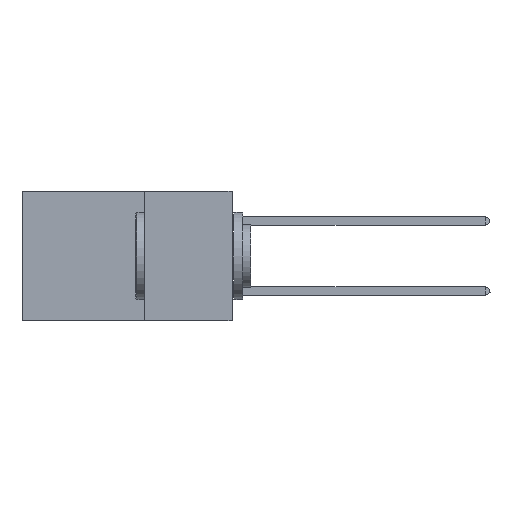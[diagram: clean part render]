
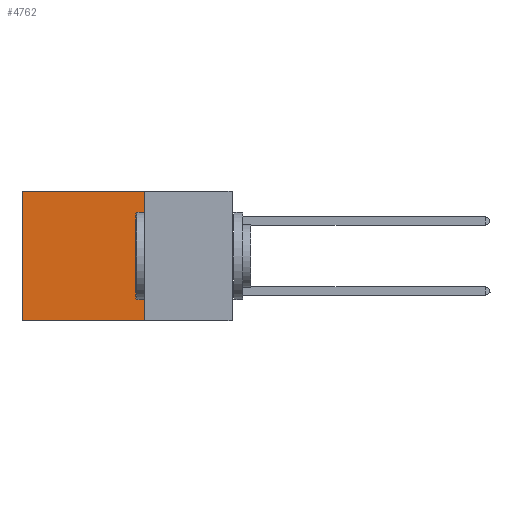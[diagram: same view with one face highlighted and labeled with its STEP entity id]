
A CAD part, left-side view. The second image highlights one B-rep face of the part: STEP entity #4762.
In plain terms, the highlighted planar face has unit normal (-1, 0, 0).
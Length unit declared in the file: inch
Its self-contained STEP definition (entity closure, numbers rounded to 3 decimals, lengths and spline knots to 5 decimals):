
#430 = VECTOR ( 'NONE', #8802, 39.37008 ) ;
#1242 = LINE ( 'NONE', #15329, #17716 ) ;
#1380 = DIRECTION ( 'NONE',  ( 0., 1., 0. ) ) ;
#1660 = DIRECTION ( 'NONE',  ( 0., 0., -1. ) ) ;
#2346 = CARTESIAN_POINT ( 'NONE',  ( 0.2875, 0.6, 0. ) ) ;
#2479 = ORIENTED_EDGE ( 'NONE', *, *, #14017, .T. ) ;
#4374 = CARTESIAN_POINT ( 'NONE',  ( 0.2875, 0.6, -0.37 ) ) ;
#4662 = AXIS2_PLACEMENT_3D ( 'NONE', #23682, #25618, #19471 ) ;
#4762 = ADVANCED_FACE ( 'NONE', ( #19505 ), #15583, .F. ) ;
#5738 = EDGE_CURVE ( 'NONE', #18091, #20064, #22649, .T. ) ;
#6403 = ORIENTED_EDGE ( 'NONE', *, *, #22559, .T. ) ;
#8564 = LINE ( 'NONE', #21800, #10503 ) ;
#8802 = DIRECTION ( 'NONE',  ( 0., 0., -1. ) ) ;
#10503 = VECTOR ( 'NONE', #1660, 39.37008 ) ;
#11326 = ORIENTED_EDGE ( 'NONE', *, *, #24099, .F. ) ;
#14017 = EDGE_CURVE ( 'NONE', #19456, #25180, #8564, .T. ) ;
#14336 = ORIENTED_EDGE ( 'NONE', *, *, #5738, .F. ) ;
#15314 = EDGE_LOOP ( 'NONE', ( #2479, #11326, #14336, #6403 ) ) ;
#15329 = CARTESIAN_POINT ( 'NONE',  ( 0.2875, 0.25, 0. ) ) ;
#15583 = PLANE ( 'NONE',  #4662 ) ;
#17716 = VECTOR ( 'NONE', #25544, 39.37008 ) ;
#18091 = VERTEX_POINT ( 'NONE', #20521 ) ;
#19456 = VERTEX_POINT ( 'NONE', #2346 ) ;
#19471 = DIRECTION ( 'NONE',  ( 0., 0., -1. ) ) ;
#19505 = FACE_OUTER_BOUND ( 'NONE', #15314, .T. ) ;
#20064 = VERTEX_POINT ( 'NONE', #23119 ) ;
#20521 = CARTESIAN_POINT ( 'NONE',  ( 0.2875, 0.25, 0. ) ) ;
#21800 = CARTESIAN_POINT ( 'NONE',  ( 0.2875, 0.6, 0. ) ) ;
#22106 = VECTOR ( 'NONE', #1380, 39.37008 ) ;
#22559 = EDGE_CURVE ( 'NONE', #18091, #19456, #1242, .T. ) ;
#22649 = LINE ( 'NONE', #23114, #430 ) ;
#23114 = CARTESIAN_POINT ( 'NONE',  ( 0.2875, 0.25, 0. ) ) ;
#23119 = CARTESIAN_POINT ( 'NONE',  ( 0.2875, 0.25, -0.37 ) ) ;
#23376 = CARTESIAN_POINT ( 'NONE',  ( 0.2875, 0.25, -0.37 ) ) ;
#23682 = CARTESIAN_POINT ( 'NONE',  ( 0.2875, 0.25, 0. ) ) ;
#24099 = EDGE_CURVE ( 'NONE', #20064, #25180, #24929, .T. ) ;
#24929 = LINE ( 'NONE', #23376, #22106 ) ;
#25180 = VERTEX_POINT ( 'NONE', #4374 ) ;
#25544 = DIRECTION ( 'NONE',  ( 0., 1., 0. ) ) ;
#25618 = DIRECTION ( 'NONE',  ( 1., 0., 0. ) ) ;
